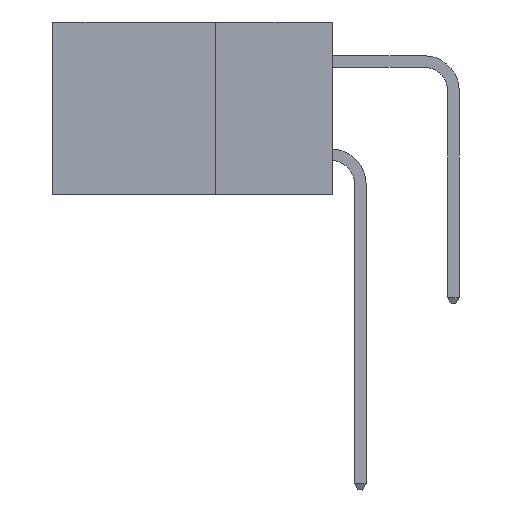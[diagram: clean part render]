
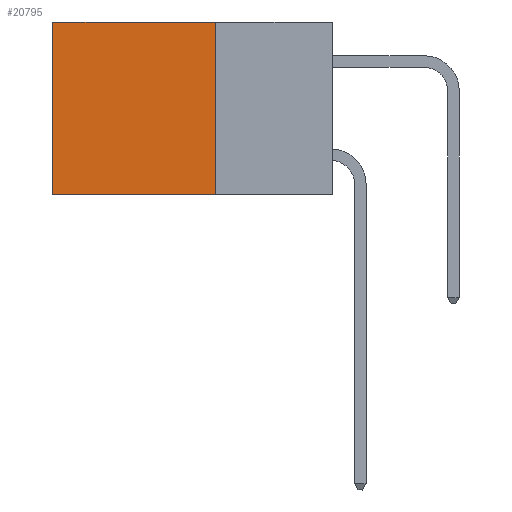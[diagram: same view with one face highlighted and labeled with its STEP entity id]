
A CAD part, left-side view. The second image highlights one B-rep face of the part: STEP entity #20795.
In plain terms, the highlighted planar face has unit normal (-1, 0, 0).
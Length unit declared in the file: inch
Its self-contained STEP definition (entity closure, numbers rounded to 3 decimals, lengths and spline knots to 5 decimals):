
#449 = ORIENTED_EDGE ( 'NONE', *, *, #27999, .F. ) ;
#857 = EDGE_CURVE ( 'NONE', #28773, #23906, #14463, .T. ) ;
#2974 = VECTOR ( 'NONE', #33605, 39.37008 ) ;
#4523 = CARTESIAN_POINT ( 'NONE',  ( 0.298, 0.6, 0. ) ) ;
#6910 = DIRECTION ( 'NONE',  ( 0., 0., -1. ) ) ;
#6943 = VERTEX_POINT ( 'NONE', #25380 ) ;
#7463 = LINE ( 'NONE', #15554, #2974 ) ;
#9248 = DIRECTION ( 'NONE',  ( 0., 1., 0. ) ) ;
#9690 = LINE ( 'NONE', #30603, #15772 ) ;
#13170 = PLANE ( 'NONE',  #27660 ) ;
#14463 = LINE ( 'NONE', #4523, #29953 ) ;
#15023 = CARTESIAN_POINT ( 'NONE',  ( 0.298, 0.25, -0.37 ) ) ;
#15554 = CARTESIAN_POINT ( 'NONE',  ( 0.298, 0.25, -0.37 ) ) ;
#15772 = VECTOR ( 'NONE', #20454, 39.37008 ) ;
#17768 = EDGE_CURVE ( 'NONE', #23939, #23906, #7463, .T. ) ;
#18393 = DIRECTION ( 'NONE',  ( 1., 0., 0. ) ) ;
#18710 = LINE ( 'NONE', #24787, #24817 ) ;
#20454 = DIRECTION ( 'NONE',  ( 0., 0., -1. ) ) ;
#20795 = ADVANCED_FACE ( 'NONE', ( #23120 ), #13170, .F. ) ;
#21102 = DIRECTION ( 'NONE',  ( 0., 0., -1. ) ) ;
#22211 = CARTESIAN_POINT ( 'NONE',  ( 0.298, 0.6, -0.37 ) ) ;
#22573 = ORIENTED_EDGE ( 'NONE', *, *, #32122, .T. ) ;
#23095 = CARTESIAN_POINT ( 'NONE',  ( 0.298, 0.6, 0. ) ) ;
#23120 = FACE_OUTER_BOUND ( 'NONE', #29175, .T. ) ;
#23906 = VERTEX_POINT ( 'NONE', #22211 ) ;
#23939 = VERTEX_POINT ( 'NONE', #15023 ) ;
#24787 = CARTESIAN_POINT ( 'NONE',  ( 0.298, 0.25, 0. ) ) ;
#24817 = VECTOR ( 'NONE', #9248, 39.37008 ) ;
#25380 = CARTESIAN_POINT ( 'NONE',  ( 0.298, 0.25, 0. ) ) ;
#26686 = ORIENTED_EDGE ( 'NONE', *, *, #857, .T. ) ;
#27357 = ORIENTED_EDGE ( 'NONE', *, *, #17768, .F. ) ;
#27660 = AXIS2_PLACEMENT_3D ( 'NONE', #31255, #18393, #21102 ) ;
#27999 = EDGE_CURVE ( 'NONE', #6943, #23939, #9690, .T. ) ;
#28773 = VERTEX_POINT ( 'NONE', #23095 ) ;
#29175 = EDGE_LOOP ( 'NONE', ( #26686, #27357, #449, #22573 ) ) ;
#29953 = VECTOR ( 'NONE', #6910, 39.37008 ) ;
#30603 = CARTESIAN_POINT ( 'NONE',  ( 0.298, 0.25, 0. ) ) ;
#31255 = CARTESIAN_POINT ( 'NONE',  ( 0.298, 0.25, 0. ) ) ;
#32122 = EDGE_CURVE ( 'NONE', #6943, #28773, #18710, .T. ) ;
#33605 = DIRECTION ( 'NONE',  ( 0., 1., 0. ) ) ;
